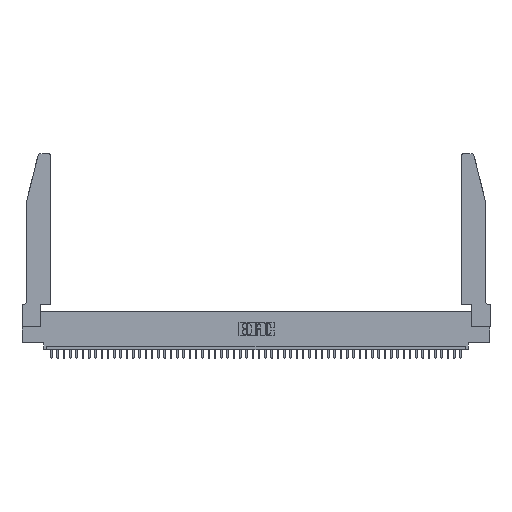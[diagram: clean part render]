
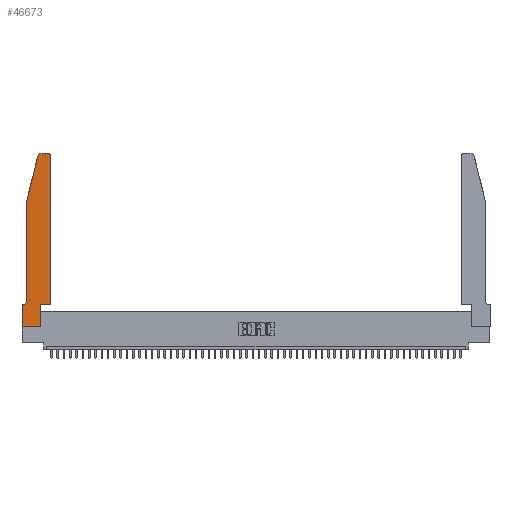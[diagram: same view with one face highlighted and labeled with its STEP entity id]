
A CAD part, top view. The second image highlights one B-rep face of the part: STEP entity #46673.
In plain terms, the highlighted planar face has unit normal (0, 0, 1).
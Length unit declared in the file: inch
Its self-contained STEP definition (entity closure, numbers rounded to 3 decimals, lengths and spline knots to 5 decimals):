
#75 = EDGE_CURVE ( 'NONE', #33316, #6303, #39247, .T. ) ;
#836 = EDGE_CURVE ( 'NONE', #41589, #11060, #29285, .T. ) ;
#1244 = CARTESIAN_POINT ( 'NONE',  ( 0.4505, 0.35, 0.37 ) ) ;
#2217 = ORIENTED_EDGE ( 'NONE', *, *, #19004, .T. ) ;
#2299 = EDGE_CURVE ( 'NONE', #30962, #35836, #18608, .T. ) ;
#2418 = CARTESIAN_POINT ( 'NONE',  ( 0.0755, 0.42, 0.37 ) ) ;
#4148 = CARTESIAN_POINT ( 'NONE',  ( 0.4205, 2.75, 0.37 ) ) ;
#4972 = VERTEX_POINT ( 'NONE', #23565 ) ;
#5454 = DIRECTION ( 'NONE',  ( -0.239, -0.971, 0. ) ) ;
#5498 = VECTOR ( 'NONE', #22182, 39.37008 ) ;
#5926 = EDGE_CURVE ( 'NONE', #39999, #11277, #9210, .T. ) ;
#6016 = DIRECTION ( 'NONE',  ( 1., 0., 0. ) ) ;
#6122 = CIRCLE ( 'NONE', #22731, 0.03 ) ;
#6274 = DIRECTION ( 'NONE',  ( 0., 1., 0. ) ) ;
#6303 = VERTEX_POINT ( 'NONE', #10521 ) ;
#6425 = VECTOR ( 'NONE', #37310, 39.37008 ) ;
#7393 = VECTOR ( 'NONE', #49976, 39.37008 ) ;
#7807 = ORIENTED_EDGE ( 'NONE', *, *, #26452, .T. ) ;
#7810 = LINE ( 'NONE', #47381, #9645 ) ;
#9210 = LINE ( 'NONE', #25795, #7393 ) ;
#9645 = VECTOR ( 'NONE', #5454, 39.37008 ) ;
#10227 = EDGE_CURVE ( 'NONE', #38441, #41589, #7810, .T. ) ;
#10521 = CARTESIAN_POINT ( 'NONE',  ( 0.284, 2.75, 0.37 ) ) ;
#10726 = CARTESIAN_POINT ( 'NONE',  ( 0.4205, 2.72, 0.37 ) ) ;
#11060 = VERTEX_POINT ( 'NONE', #2418 ) ;
#11277 = VERTEX_POINT ( 'NONE', #17340 ) ;
#11446 = CIRCLE ( 'NONE', #35367, 0.03 ) ;
#11460 = ORIENTED_EDGE ( 'NONE', *, *, #48166, .T. ) ;
#12291 = DIRECTION ( 'NONE',  ( 1., 0., 0. ) ) ;
#12970 = CARTESIAN_POINT ( 'NONE',  ( 0.2865, 0., 0.37 ) ) ;
#13349 = PLANE ( 'NONE',  #45372 ) ;
#14328 = EDGE_CURVE ( 'NONE', #40157, #4972, #26610, .T. ) ;
#16306 = ORIENTED_EDGE ( 'NONE', *, *, #17197, .T. ) ;
#16793 = LINE ( 'NONE', #40361, #47166 ) ;
#17197 = EDGE_CURVE ( 'NONE', #6303, #38441, #6122, .T. ) ;
#17340 = CARTESIAN_POINT ( 'NONE',  ( 0.2865, 0.35, 0.37 ) ) ;
#18608 = LINE ( 'NONE', #26058, #29825 ) ;
#19004 = EDGE_CURVE ( 'NONE', #35836, #33316, #11446, .T. ) ;
#20226 = CARTESIAN_POINT ( 'NONE',  ( 0.0755, 2., 0.37 ) ) ;
#20309 = EDGE_CURVE ( 'NONE', #11060, #26024, #24397, .T. ) ;
#20500 = DIRECTION ( 'NONE',  ( 0., -1., 0. ) ) ;
#21021 = CARTESIAN_POINT ( 'NONE',  ( 0.0755, 2., 0.37 ) ) ;
#22182 = DIRECTION ( 'NONE',  ( 0., -1., 0. ) ) ;
#22593 = CARTESIAN_POINT ( 'NONE',  ( 0.0055, 0.42, 0.37 ) ) ;
#22731 = AXIS2_PLACEMENT_3D ( 'NONE', #29779, #37699, #6016 ) ;
#23231 = DIRECTION ( 'NONE',  ( 0., 0., 1. ) ) ;
#23565 = CARTESIAN_POINT ( 'NONE',  ( 0., 0., 0.37 ) ) ;
#24397 = CIRCLE ( 'NONE', #45409, 0.07 ) ;
#24751 = ORIENTED_EDGE ( 'NONE', *, *, #2299, .T. ) ;
#25190 = DIRECTION ( 'NONE',  ( 0., 0., 1. ) ) ;
#25636 = CARTESIAN_POINT ( 'NONE',  ( 0.2605, 2.75, 0.37 ) ) ;
#25795 = CARTESIAN_POINT ( 'NONE',  ( 0.2865, 0.35, 0.37 ) ) ;
#26024 = VERTEX_POINT ( 'NONE', #46461 ) ;
#26058 = CARTESIAN_POINT ( 'NONE',  ( 0.4505, 0.35, 0.37 ) ) ;
#26452 = EDGE_CURVE ( 'NONE', #11277, #30962, #40082, .T. ) ;
#26583 = DIRECTION ( 'NONE',  ( 0., 0., -1. ) ) ;
#26610 = LINE ( 'NONE', #37418, #5498 ) ;
#27091 = ORIENTED_EDGE ( 'NONE', *, *, #14328, .T. ) ;
#28337 = ORIENTED_EDGE ( 'NONE', *, *, #5926, .T. ) ;
#28452 = ORIENTED_EDGE ( 'NONE', *, *, #30312, .T. ) ;
#28831 = CARTESIAN_POINT ( 'NONE',  ( 0.25487, 2.72718, 0.37 ) ) ;
#29285 = LINE ( 'NONE', #21021, #39773 ) ;
#29779 = CARTESIAN_POINT ( 'NONE',  ( 0.284, 2.72, 0.37 ) ) ;
#29825 = VECTOR ( 'NONE', #6274, 39.37008 ) ;
#30312 = EDGE_CURVE ( 'NONE', #4972, #39999, #16793, .T. ) ;
#30784 = DIRECTION ( 'NONE',  ( 1., 0., 0. ) ) ;
#30962 = VERTEX_POINT ( 'NONE', #1244 ) ;
#31335 = CARTESIAN_POINT ( 'NONE',  ( 0., 0.35, 0.37 ) ) ;
#32116 = LINE ( 'NONE', #41608, #38308 ) ;
#32950 = CARTESIAN_POINT ( 'NONE',  ( 0., 0.35, 0.37 ) ) ;
#33092 = ORIENTED_EDGE ( 'NONE', *, *, #75, .T. ) ;
#33316 = VERTEX_POINT ( 'NONE', #4148 ) ;
#34354 = ORIENTED_EDGE ( 'NONE', *, *, #20309, .T. ) ;
#35145 = ORIENTED_EDGE ( 'NONE', *, *, #836, .T. ) ;
#35183 = ORIENTED_EDGE ( 'NONE', *, *, #10227, .T. ) ;
#35367 = AXIS2_PLACEMENT_3D ( 'NONE', #10726, #23231, #35806 ) ;
#35806 = DIRECTION ( 'NONE',  ( 1., 0., 0. ) ) ;
#35836 = VERTEX_POINT ( 'NONE', #46419 ) ;
#37310 = DIRECTION ( 'NONE',  ( -1., 0., 0. ) ) ;
#37418 = CARTESIAN_POINT ( 'NONE',  ( 0., 0., 0.37 ) ) ;
#37699 = DIRECTION ( 'NONE',  ( 0., 0., 1. ) ) ;
#38308 = VECTOR ( 'NONE', #45775, 39.37008 ) ;
#38441 = VERTEX_POINT ( 'NONE', #28831 ) ;
#39247 = LINE ( 'NONE', #25636, #6425 ) ;
#39773 = VECTOR ( 'NONE', #20500, 39.37008 ) ;
#39999 = VERTEX_POINT ( 'NONE', #12970 ) ;
#40082 = LINE ( 'NONE', #50515, #43856 ) ;
#40157 = VERTEX_POINT ( 'NONE', #31335 ) ;
#40361 = CARTESIAN_POINT ( 'NONE',  ( 0., 0., 0.37 ) ) ;
#41075 = DIRECTION ( 'NONE',  ( 1., 0., 0. ) ) ;
#41589 = VERTEX_POINT ( 'NONE', #20226 ) ;
#41608 = CARTESIAN_POINT ( 'NONE',  ( 0.0755, 0.35, 0.37 ) ) ;
#43856 = VECTOR ( 'NONE', #30784, 39.37008 ) ;
#45372 = AXIS2_PLACEMENT_3D ( 'NONE', #32950, #25190, #41075 ) ;
#45409 = AXIS2_PLACEMENT_3D ( 'NONE', #22593, #26583, #50111 ) ;
#45775 = DIRECTION ( 'NONE',  ( -1., 0., 0. ) ) ;
#46419 = CARTESIAN_POINT ( 'NONE',  ( 0.4505, 2.72, 0.37 ) ) ;
#46461 = CARTESIAN_POINT ( 'NONE',  ( 0.0055, 0.35, 0.37 ) ) ;
#46673 = ADVANCED_FACE ( 'NONE', ( #48041 ), #13349, .T. ) ;
#47166 = VECTOR ( 'NONE', #12291, 39.37008 ) ;
#47381 = CARTESIAN_POINT ( 'NONE',  ( 0.0755, 2., 0.37 ) ) ;
#48041 = FACE_OUTER_BOUND ( 'NONE', #48958, .T. ) ;
#48166 = EDGE_CURVE ( 'NONE', #26024, #40157, #32116, .T. ) ;
#48958 = EDGE_LOOP ( 'NONE', ( #33092, #16306, #35183, #35145, #34354, #11460, #27091, #28452, #28337, #7807, #24751, #2217 ) ) ;
#49976 = DIRECTION ( 'NONE',  ( 0., 1., 0. ) ) ;
#50111 = DIRECTION ( 'NONE',  ( -1., 0., 0. ) ) ;
#50515 = CARTESIAN_POINT ( 'NONE',  ( 0.4505, 0.35, 0.37 ) ) ;
